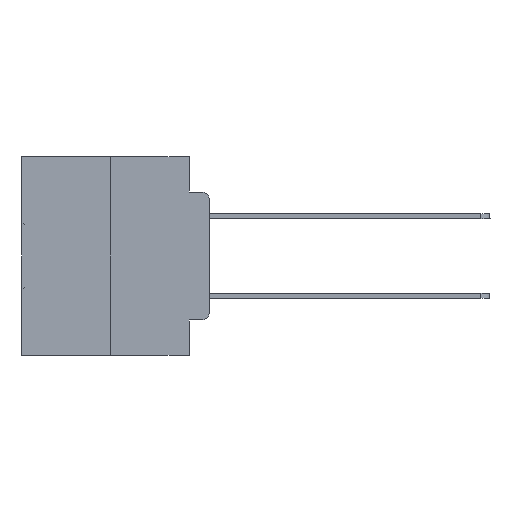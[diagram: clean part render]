
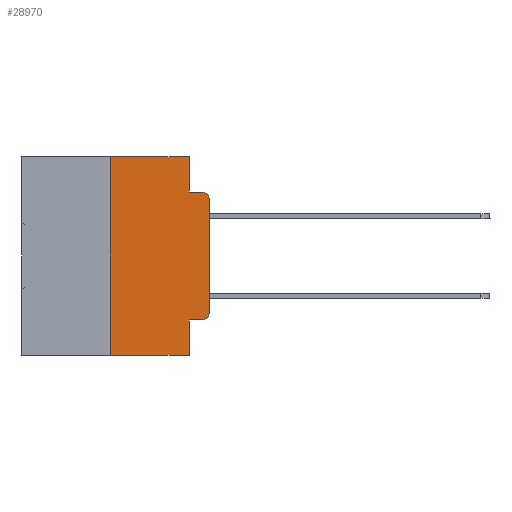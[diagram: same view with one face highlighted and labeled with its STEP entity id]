
A CAD part, left-side view. The second image highlights one B-rep face of the part: STEP entity #28970.
In plain terms, the highlighted planar face has unit normal (-1, 0, 0).
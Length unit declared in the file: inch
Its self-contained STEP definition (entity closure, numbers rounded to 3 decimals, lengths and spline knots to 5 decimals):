
#416 = VECTOR ( 'NONE', #10753, 39.37008 ) ;
#447 = VERTEX_POINT ( 'NONE', #3742 ) ;
#1001 = CARTESIAN_POINT ( 'NONE',  ( 0., 0.051, 0. ) ) ;
#2106 = LINE ( 'NONE', #2446, #24708 ) ;
#2239 = VECTOR ( 'NONE', #21877, 39.37008 ) ;
#2358 = CARTESIAN_POINT ( 'NONE',  ( 0., 0.051, 0. ) ) ;
#2446 = CARTESIAN_POINT ( 'NONE',  ( 0., 0.25, 0. ) ) ;
#3058 = CARTESIAN_POINT ( 'NONE',  ( 0., 0., 0. ) ) ;
#3274 = ORIENTED_EDGE ( 'NONE', *, *, #33162, .F. ) ;
#3742 = CARTESIAN_POINT ( 'NONE',  ( 0., 0., -0.3915 ) ) ;
#4144 = VERTEX_POINT ( 'NONE', #7498 ) ;
#4231 = CARTESIAN_POINT ( 'NONE',  ( 0., 0.051, 0. ) ) ;
#4339 = DIRECTION ( 'NONE',  ( 0., 0., -1. ) ) ;
#5239 = EDGE_CURVE ( 'NONE', #5948, #8341, #27159, .T. ) ;
#5691 = ORIENTED_EDGE ( 'NONE', *, *, #21122, .T. ) ;
#5907 = DIRECTION ( 'NONE',  ( 0., 0., -1. ) ) ;
#5948 = VERTEX_POINT ( 'NONE', #1001 ) ;
#6074 = ORIENTED_EDGE ( 'NONE', *, *, #12158, .T. ) ;
#6088 = EDGE_LOOP ( 'NONE', ( #6074, #13637, #23343, #29091, #3274, #24783, #33416, #27786, #5691, #18051 ) ) ;
#6375 = CARTESIAN_POINT ( 'NONE',  ( 0., 0.02, -0.1085 ) ) ;
#7394 = CARTESIAN_POINT ( 'NONE',  ( 0., 0.473, 0. ) ) ;
#7498 = CARTESIAN_POINT ( 'NONE',  ( 0., 0.25, 0. ) ) ;
#7601 = EDGE_CURVE ( 'NONE', #9909, #32971, #31261, .T. ) ;
#8341 = VERTEX_POINT ( 'NONE', #12333 ) ;
#9159 = VECTOR ( 'NONE', #34209, 39.37008 ) ;
#9219 = CARTESIAN_POINT ( 'NONE',  ( 0., 0.051, -0.0885 ) ) ;
#9513 = CARTESIAN_POINT ( 'NONE',  ( 0., 0.051, -0.5 ) ) ;
#9601 = LINE ( 'NONE', #24966, #15797 ) ;
#9909 = VERTEX_POINT ( 'NONE', #29081 ) ;
#10170 = CARTESIAN_POINT ( 'NONE',  ( 0., 0.02, -0.4115 ) ) ;
#10237 = VECTOR ( 'NONE', #27865, 39.37008 ) ;
#10273 = VERTEX_POINT ( 'NONE', #30005 ) ;
#10501 = CARTESIAN_POINT ( 'NONE',  ( 0., 0.02, -0.0885 ) ) ;
#10576 = LINE ( 'NONE', #3058, #2239 ) ;
#10700 = DIRECTION ( 'NONE',  ( 0., 0., -1. ) ) ;
#10753 = DIRECTION ( 'NONE',  ( 0., -1., 0. ) ) ;
#11438 = CARTESIAN_POINT ( 'NONE',  ( 0., 0.473, -0.5 ) ) ;
#11784 = CARTESIAN_POINT ( 'NONE',  ( 0., 0.25, -0.5 ) ) ;
#11861 = DIRECTION ( 'NONE',  ( 0., -1., 0. ) ) ;
#12158 = EDGE_CURVE ( 'NONE', #447, #10273, #10576, .T. ) ;
#12333 = CARTESIAN_POINT ( 'NONE',  ( 0., 0.051, -0.0885 ) ) ;
#13550 = CARTESIAN_POINT ( 'NONE',  ( 0., 0.02, -0.3915 ) ) ;
#13637 = ORIENTED_EDGE ( 'NONE', *, *, #16627, .T. ) ;
#13715 = PLANE ( 'NONE',  #22543 ) ;
#13856 = EDGE_CURVE ( 'NONE', #21708, #4144, #2106, .T. ) ;
#15797 = VECTOR ( 'NONE', #30242, 39.37008 ) ;
#15900 = CIRCLE ( 'NONE', #33132, 0.02 ) ;
#16396 = DIRECTION ( 'NONE',  ( 1., 0., 0. ) ) ;
#16627 = EDGE_CURVE ( 'NONE', #10273, #22148, #23689, .T. ) ;
#17339 = EDGE_CURVE ( 'NONE', #21708, #32971, #21533, .T. ) ;
#18051 = ORIENTED_EDGE ( 'NONE', *, *, #19810, .T. ) ;
#19477 = VECTOR ( 'NONE', #4339, 39.37008 ) ;
#19674 = DIRECTION ( 'NONE',  ( -1., 0., 0. ) ) ;
#19810 = EDGE_CURVE ( 'NONE', #24446, #447, #15900, .T. ) ;
#20883 = LINE ( 'NONE', #9219, #24253 ) ;
#20924 = LINE ( 'NONE', #7394, #416 ) ;
#21122 = EDGE_CURVE ( 'NONE', #9909, #24446, #9601, .T. ) ;
#21533 = LINE ( 'NONE', #11438, #10237 ) ;
#21708 = VERTEX_POINT ( 'NONE', #11784 ) ;
#21877 = DIRECTION ( 'NONE',  ( 0., 0., 1. ) ) ;
#22008 = DIRECTION ( 'NONE',  ( -1., 0., 0. ) ) ;
#22148 = VERTEX_POINT ( 'NONE', #10501 ) ;
#22543 = AXIS2_PLACEMENT_3D ( 'NONE', #26757, #16396, #10700 ) ;
#22953 = AXIS2_PLACEMENT_3D ( 'NONE', #6375, #19674, #5907 ) ;
#23343 = ORIENTED_EDGE ( 'NONE', *, *, #24841, .F. ) ;
#23689 = CIRCLE ( 'NONE', #22953, 0.02 ) ;
#24253 = VECTOR ( 'NONE', #11861, 39.37008 ) ;
#24446 = VERTEX_POINT ( 'NONE', #10170 ) ;
#24708 = VECTOR ( 'NONE', #29385, 39.37008 ) ;
#24783 = ORIENTED_EDGE ( 'NONE', *, *, #13856, .F. ) ;
#24841 = EDGE_CURVE ( 'NONE', #8341, #22148, #20883, .T. ) ;
#24966 = CARTESIAN_POINT ( 'NONE',  ( 0., 0.051, -0.4115 ) ) ;
#26757 = CARTESIAN_POINT ( 'NONE',  ( 0., 0.473, 0. ) ) ;
#27157 = DIRECTION ( 'NONE',  ( 0., 0., -1. ) ) ;
#27159 = LINE ( 'NONE', #2358, #9159 ) ;
#27786 = ORIENTED_EDGE ( 'NONE', *, *, #7601, .F. ) ;
#27865 = DIRECTION ( 'NONE',  ( 0., -1., 0. ) ) ;
#28970 = ADVANCED_FACE ( 'NONE', ( #34450 ), #13715, .F. ) ;
#29081 = CARTESIAN_POINT ( 'NONE',  ( 0., 0.051, -0.4115 ) ) ;
#29091 = ORIENTED_EDGE ( 'NONE', *, *, #5239, .F. ) ;
#29385 = DIRECTION ( 'NONE',  ( 0., 0., 1. ) ) ;
#30005 = CARTESIAN_POINT ( 'NONE',  ( 0., 0., -0.1085 ) ) ;
#30242 = DIRECTION ( 'NONE',  ( 0., -1., 0. ) ) ;
#31261 = LINE ( 'NONE', #4231, #19477 ) ;
#32971 = VERTEX_POINT ( 'NONE', #9513 ) ;
#33132 = AXIS2_PLACEMENT_3D ( 'NONE', #13550, #22008, #27157 ) ;
#33162 = EDGE_CURVE ( 'NONE', #4144, #5948, #20924, .T. ) ;
#33416 = ORIENTED_EDGE ( 'NONE', *, *, #17339, .T. ) ;
#34209 = DIRECTION ( 'NONE',  ( 0., 0., -1. ) ) ;
#34450 = FACE_OUTER_BOUND ( 'NONE', #6088, .T. ) ;
